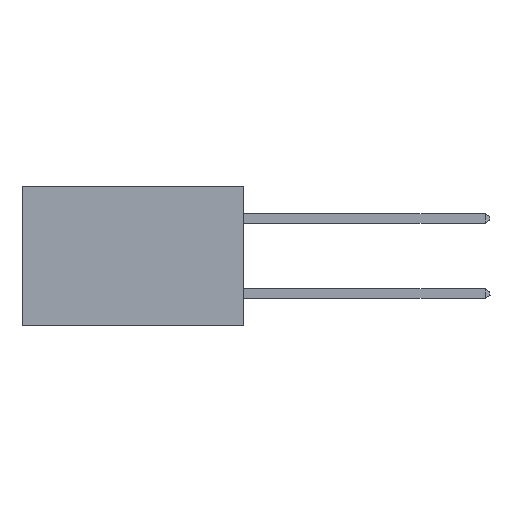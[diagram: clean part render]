
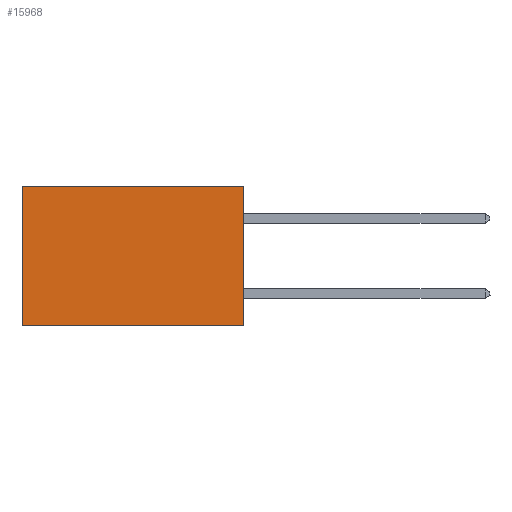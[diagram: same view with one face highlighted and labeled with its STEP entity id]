
A CAD part, left-side view. The second image highlights one B-rep face of the part: STEP entity #15968.
In plain terms, the highlighted planar face has unit normal (-1, 0, 0).
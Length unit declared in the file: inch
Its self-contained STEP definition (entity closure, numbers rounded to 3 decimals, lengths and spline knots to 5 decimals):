
#2 = CARTESIAN_POINT ( 'NONE',  ( 0.277, 0., -0.37 ) ) ;
#1073 = VERTEX_POINT ( 'NONE', #16523 ) ;
#3279 = VECTOR ( 'NONE', #11287, 39.37008 ) ;
#4926 = VERTEX_POINT ( 'NONE', #31257 ) ;
#5773 = ORIENTED_EDGE ( 'NONE', *, *, #29184, .F. ) ;
#6211 = ORIENTED_EDGE ( 'NONE', *, *, #24795, .T. ) ;
#6647 = FACE_OUTER_BOUND ( 'NONE', #23904, .T. ) ;
#6660 = CARTESIAN_POINT ( 'NONE',  ( 0.277, 0., -0.37 ) ) ;
#7205 = ORIENTED_EDGE ( 'NONE', *, *, #24838, .T. ) ;
#7698 = DIRECTION ( 'NONE',  ( 1., 0., 0. ) ) ;
#8754 = CARTESIAN_POINT ( 'NONE',  ( 0.277, 0., -0.37 ) ) ;
#11287 = DIRECTION ( 'NONE',  ( 0., 0., -1. ) ) ;
#13600 = VECTOR ( 'NONE', #21820, 39.37008 ) ;
#14198 = CARTESIAN_POINT ( 'NONE',  ( 0.277, 0., 0. ) ) ;
#15968 = ADVANCED_FACE ( 'NONE', ( #6647 ), #17725, .F. ) ;
#16523 = CARTESIAN_POINT ( 'NONE',  ( 0.277, 0.59, 0. ) ) ;
#16715 = LINE ( 'NONE', #14198, #22731 ) ;
#16719 = DIRECTION ( 'NONE',  ( 0., 1., 0. ) ) ;
#17503 = VECTOR ( 'NONE', #19059, 39.37008 ) ;
#17725 = PLANE ( 'NONE',  #20949 ) ;
#18079 = EDGE_CURVE ( 'NONE', #26981, #28588, #30708, .T. ) ;
#19059 = DIRECTION ( 'NONE',  ( 0., 0., -1. ) ) ;
#20949 = AXIS2_PLACEMENT_3D ( 'NONE', #2, #7698, #25495 ) ;
#20953 = ORIENTED_EDGE ( 'NONE', *, *, #18079, .F. ) ;
#21820 = DIRECTION ( 'NONE',  ( 0., 1., 0. ) ) ;
#21898 = LINE ( 'NONE', #8754, #3279 ) ;
#22731 = VECTOR ( 'NONE', #16719, 39.37008 ) ;
#23069 = CARTESIAN_POINT ( 'NONE',  ( 0.277, 0., -0.37 ) ) ;
#23904 = EDGE_LOOP ( 'NONE', ( #6211, #20953, #5773, #7205 ) ) ;
#24795 = EDGE_CURVE ( 'NONE', #1073, #28588, #31064, .T. ) ;
#24838 = EDGE_CURVE ( 'NONE', #4926, #1073, #16715, .T. ) ;
#25495 = DIRECTION ( 'NONE',  ( 0., 0., -1. ) ) ;
#26981 = VERTEX_POINT ( 'NONE', #23069 ) ;
#28588 = VERTEX_POINT ( 'NONE', #31834 ) ;
#29184 = EDGE_CURVE ( 'NONE', #4926, #26981, #21898, .T. ) ;
#29265 = CARTESIAN_POINT ( 'NONE',  ( 0.277, 0.59, -0.37 ) ) ;
#30708 = LINE ( 'NONE', #6660, #13600 ) ;
#31064 = LINE ( 'NONE', #29265, #17503 ) ;
#31257 = CARTESIAN_POINT ( 'NONE',  ( 0.277, 0., 0. ) ) ;
#31834 = CARTESIAN_POINT ( 'NONE',  ( 0.277, 0.59, -0.37 ) ) ;
